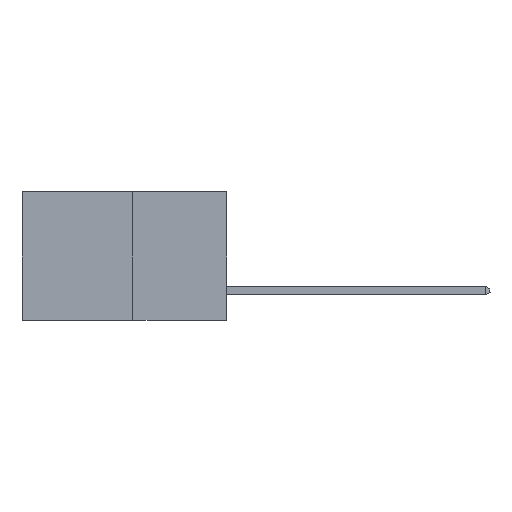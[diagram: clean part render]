
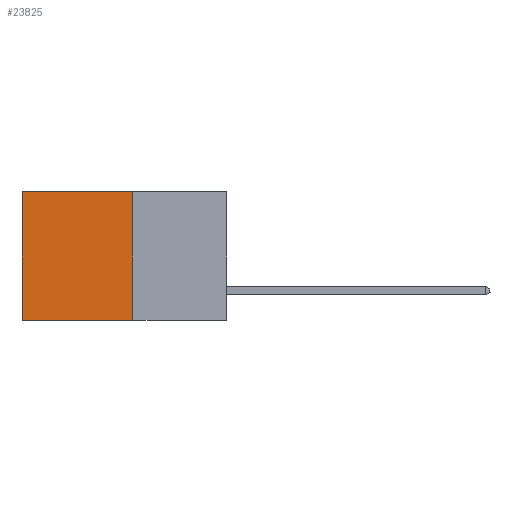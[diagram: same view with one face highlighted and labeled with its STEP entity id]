
A CAD part, left-side view. The second image highlights one B-rep face of the part: STEP entity #23825.
In plain terms, the highlighted planar face has unit normal (-1, 0, 0).
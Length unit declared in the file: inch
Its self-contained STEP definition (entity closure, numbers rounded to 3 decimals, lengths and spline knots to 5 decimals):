
#257 = LINE ( 'NONE', #3549, #21678 ) ;
#2144 = EDGE_CURVE ( 'NONE', #7313, #24068, #28755, .T. ) ;
#2393 = AXIS2_PLACEMENT_3D ( 'NONE', #16333, #8911, #26262 ) ;
#2754 = CARTESIAN_POINT ( 'NONE',  ( 0.277, 0.27, -0.37 ) ) ;
#3549 = CARTESIAN_POINT ( 'NONE',  ( 0.277, 0.59, -0.37 ) ) ;
#4508 = ORIENTED_EDGE ( 'NONE', *, *, #23069, .T. ) ;
#6353 = DIRECTION ( 'NONE',  ( 0., 1., 0. ) ) ;
#7313 = VERTEX_POINT ( 'NONE', #26678 ) ;
#7656 = ORIENTED_EDGE ( 'NONE', *, *, #28311, .T. ) ;
#7799 = CARTESIAN_POINT ( 'NONE',  ( 0.277, 0.27, -0.37 ) ) ;
#8911 = DIRECTION ( 'NONE',  ( 1., 0., 0. ) ) ;
#11279 = CARTESIAN_POINT ( 'NONE',  ( 0.277, 0.27, -0.37 ) ) ;
#11363 = DIRECTION ( 'NONE',  ( 0., 0., -1. ) ) ;
#14192 = EDGE_LOOP ( 'NONE', ( #4508, #17284, #19178, #7656 ) ) ;
#14808 = VERTEX_POINT ( 'NONE', #19005 ) ;
#16333 = CARTESIAN_POINT ( 'NONE',  ( 0.277, 0.27, -0.37 ) ) ;
#17284 = ORIENTED_EDGE ( 'NONE', *, *, #19105, .F. ) ;
#19005 = CARTESIAN_POINT ( 'NONE',  ( 0.277, 0.59, -0.37 ) ) ;
#19105 = EDGE_CURVE ( 'NONE', #24068, #14808, #28797, .T. ) ;
#19178 = ORIENTED_EDGE ( 'NONE', *, *, #2144, .F. ) ;
#20049 = LINE ( 'NONE', #23769, #25846 ) ;
#20122 = DIRECTION ( 'NONE',  ( 0., 1., 0. ) ) ;
#20234 = VERTEX_POINT ( 'NONE', #28594 ) ;
#21483 = VECTOR ( 'NONE', #11363, 39.37008 ) ;
#21678 = VECTOR ( 'NONE', #25983, 39.37008 ) ;
#22309 = VECTOR ( 'NONE', #20122, 39.37008 ) ;
#22417 = FACE_OUTER_BOUND ( 'NONE', #14192, .T. ) ;
#23069 = EDGE_CURVE ( 'NONE', #20234, #14808, #257, .T. ) ;
#23769 = CARTESIAN_POINT ( 'NONE',  ( 0.277, 0.27, 0. ) ) ;
#23796 = PLANE ( 'NONE',  #2393 ) ;
#23825 = ADVANCED_FACE ( 'NONE', ( #22417 ), #23796, .F. ) ;
#24068 = VERTEX_POINT ( 'NONE', #7799 ) ;
#25846 = VECTOR ( 'NONE', #6353, 39.37008 ) ;
#25983 = DIRECTION ( 'NONE',  ( 0., 0., -1. ) ) ;
#26262 = DIRECTION ( 'NONE',  ( 0., 0., -1. ) ) ;
#26678 = CARTESIAN_POINT ( 'NONE',  ( 0.277, 0.27, 0. ) ) ;
#28311 = EDGE_CURVE ( 'NONE', #7313, #20234, #20049, .T. ) ;
#28594 = CARTESIAN_POINT ( 'NONE',  ( 0.277, 0.59, 0. ) ) ;
#28755 = LINE ( 'NONE', #11279, #21483 ) ;
#28797 = LINE ( 'NONE', #2754, #22309 ) ;
